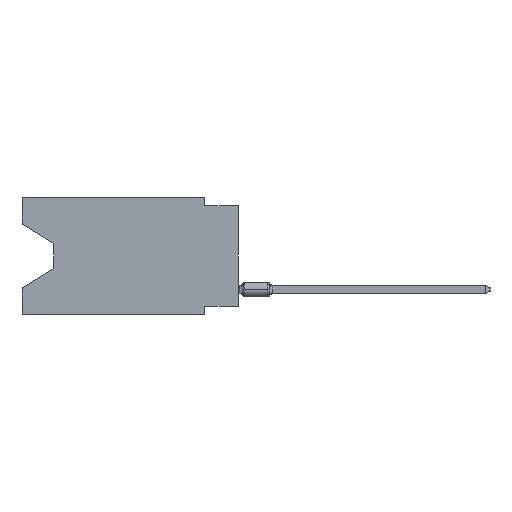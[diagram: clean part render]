
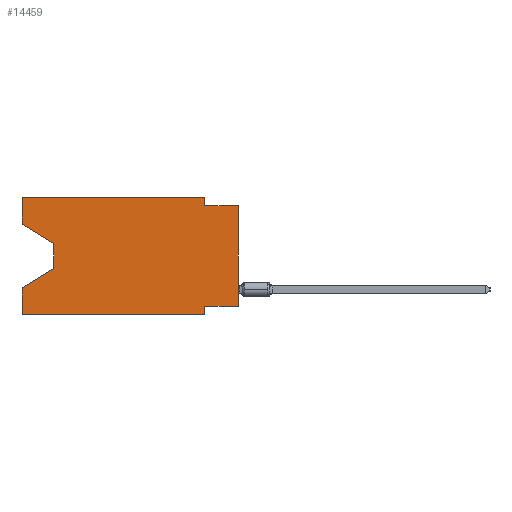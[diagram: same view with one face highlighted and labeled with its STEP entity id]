
A CAD part, left-side view. The second image highlights one B-rep face of the part: STEP entity #14459.
In plain terms, the highlighted planar face has unit normal (-1, 0, 0).
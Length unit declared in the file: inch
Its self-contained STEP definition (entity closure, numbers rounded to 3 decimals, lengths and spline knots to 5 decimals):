
#337 = CARTESIAN_POINT ( 'NONE',  ( 0., 0., -0.325 ) ) ;
#362 = VERTEX_POINT ( 'NONE', #9752 ) ;
#591 = VECTOR ( 'NONE', #44766, 39.37008 ) ;
#774 = CARTESIAN_POINT ( 'NONE',  ( 0., 0., -0.025 ) ) ;
#1442 = VECTOR ( 'NONE', #28018, 39.37008 ) ;
#1944 = ORIENTED_EDGE ( 'NONE', *, *, #45231, .F. ) ;
#2116 = AXIS2_PLACEMENT_3D ( 'NONE', #19843, #26603, #19621 ) ;
#2626 = VECTOR ( 'NONE', #33561, 39.37008 ) ;
#2819 = CARTESIAN_POINT ( 'NONE',  ( 0., 0.55, -0.138 ) ) ;
#3111 = ORIENTED_EDGE ( 'NONE', *, *, #26952, .F. ) ;
#3164 = VECTOR ( 'NONE', #10045, 39.37008 ) ;
#3752 = VERTEX_POINT ( 'NONE', #2819 ) ;
#5478 = ORIENTED_EDGE ( 'NONE', *, *, #40835, .T. ) ;
#5679 = PLANE ( 'NONE',  #2116 ) ;
#6132 = FACE_OUTER_BOUND ( 'NONE', #6671, .T. ) ;
#6144 = CARTESIAN_POINT ( 'NONE',  ( 0., 0., 0. ) ) ;
#6322 = EDGE_CURVE ( 'NONE', #36240, #7142, #17502, .T. ) ;
#6671 = EDGE_LOOP ( 'NONE', ( #13034, #44994, #35203, #3111, #5478, #38925, #16102, #21252, #15470, #29379, #1944, #29011 ) ) ;
#7032 = VERTEX_POINT ( 'NONE', #10753 ) ;
#7142 = VERTEX_POINT ( 'NONE', #774 ) ;
#7881 = VECTOR ( 'NONE', #20769, 39.37008 ) ;
#8308 = LINE ( 'NONE', #36684, #13672 ) ;
#8910 = CARTESIAN_POINT ( 'NONE',  ( 0., 0.55, -0.138 ) ) ;
#9699 = CARTESIAN_POINT ( 'NONE',  ( 0., 0.1, 0. ) ) ;
#9752 = CARTESIAN_POINT ( 'NONE',  ( 0., 0.645, -0.35 ) ) ;
#10045 = DIRECTION ( 'NONE',  ( 0., 0.855, -0.519 ) ) ;
#10753 = CARTESIAN_POINT ( 'NONE',  ( 0., 0.1, -0.025 ) ) ;
#10934 = LINE ( 'NONE', #37156, #29182 ) ;
#10950 = VECTOR ( 'NONE', #18762, 39.37008 ) ;
#11031 = DIRECTION ( 'NONE',  ( 0., 0., 1. ) ) ;
#11550 = LINE ( 'NONE', #29010, #10950 ) ;
#12485 = DIRECTION ( 'NONE',  ( 0., 0., -1. ) ) ;
#13034 = ORIENTED_EDGE ( 'NONE', *, *, #34110, .T. ) ;
#13130 = EDGE_CURVE ( 'NONE', #15213, #35680, #25217, .T. ) ;
#13624 = CARTESIAN_POINT ( 'NONE',  ( 0., 0.645, -0.35 ) ) ;
#13672 = VECTOR ( 'NONE', #25984, 39.37008 ) ;
#14065 = CARTESIAN_POINT ( 'NONE',  ( 0., 0., -0.325 ) ) ;
#14459 = ADVANCED_FACE ( 'NONE', ( #6132 ), #5679, .F. ) ;
#15177 = LINE ( 'NONE', #8910, #2626 ) ;
#15213 = VERTEX_POINT ( 'NONE', #26420 ) ;
#15470 = ORIENTED_EDGE ( 'NONE', *, *, #18663, .F. ) ;
#16076 = LINE ( 'NONE', #44230, #25822 ) ;
#16102 = ORIENTED_EDGE ( 'NONE', *, *, #35900, .F. ) ;
#17017 = LINE ( 'NONE', #27714, #3164 ) ;
#17502 = LINE ( 'NONE', #6144, #7881 ) ;
#18159 = CARTESIAN_POINT ( 'NONE',  ( 0., 0.1, -0.35 ) ) ;
#18237 = LINE ( 'NONE', #14065, #1442 ) ;
#18663 = EDGE_CURVE ( 'NONE', #7032, #7142, #8308, .T. ) ;
#18728 = VECTOR ( 'NONE', #11031, 39.37008 ) ;
#18762 = DIRECTION ( 'NONE',  ( 0., -0.855, -0.519 ) ) ;
#18986 = CARTESIAN_POINT ( 'NONE',  ( 0., 0.645, 0. ) ) ;
#19104 = DIRECTION ( 'NONE',  ( 0., -1., 0. ) ) ;
#19621 = DIRECTION ( 'NONE',  ( 0., 0., -1. ) ) ;
#19843 = CARTESIAN_POINT ( 'NONE',  ( 0., 0.645, 0. ) ) ;
#20078 = VERTEX_POINT ( 'NONE', #23554 ) ;
#20769 = DIRECTION ( 'NONE',  ( 0., 0., 1. ) ) ;
#21252 = ORIENTED_EDGE ( 'NONE', *, *, #6322, .T. ) ;
#23001 = VECTOR ( 'NONE', #28398, 39.37008 ) ;
#23168 = EDGE_CURVE ( 'NONE', #30504, #20078, #17017, .T. ) ;
#23554 = CARTESIAN_POINT ( 'NONE',  ( 0., 0.645, -0.26975 ) ) ;
#25217 = LINE ( 'NONE', #29391, #18728 ) ;
#25822 = VECTOR ( 'NONE', #19104, 39.37008 ) ;
#25984 = DIRECTION ( 'NONE',  ( 0., -1., 0. ) ) ;
#26420 = CARTESIAN_POINT ( 'NONE',  ( 0., 0.645, -0.08025 ) ) ;
#26512 = CARTESIAN_POINT ( 'NONE',  ( 0., 0.55, -0.212 ) ) ;
#26603 = DIRECTION ( 'NONE',  ( 1., 0., 0. ) ) ;
#26952 = EDGE_CURVE ( 'NONE', #362, #20078, #30561, .T. ) ;
#27352 = LINE ( 'NONE', #13624, #33669 ) ;
#27714 = CARTESIAN_POINT ( 'NONE',  ( 0., 0.55, -0.212 ) ) ;
#28018 = DIRECTION ( 'NONE',  ( 0., 1., 0. ) ) ;
#28398 = DIRECTION ( 'NONE',  ( 0., 0., -1. ) ) ;
#29010 = CARTESIAN_POINT ( 'NONE',  ( 0., 0.645, -0.08025 ) ) ;
#29011 = ORIENTED_EDGE ( 'NONE', *, *, #13130, .F. ) ;
#29182 = VECTOR ( 'NONE', #12485, 39.37008 ) ;
#29379 = ORIENTED_EDGE ( 'NONE', *, *, #40695, .F. ) ;
#29391 = CARTESIAN_POINT ( 'NONE',  ( 0., 0.645, 0. ) ) ;
#30504 = VERTEX_POINT ( 'NONE', #26512 ) ;
#30561 = LINE ( 'NONE', #45226, #591 ) ;
#31239 = EDGE_CURVE ( 'NONE', #3752, #30504, #15177, .T. ) ;
#31698 = CARTESIAN_POINT ( 'NONE',  ( 0., 0.1, -0.325 ) ) ;
#33561 = DIRECTION ( 'NONE',  ( 0., 0., -1. ) ) ;
#33669 = VECTOR ( 'NONE', #41095, 39.37008 ) ;
#34110 = EDGE_CURVE ( 'NONE', #15213, #3752, #11550, .T. ) ;
#35203 = ORIENTED_EDGE ( 'NONE', *, *, #23168, .T. ) ;
#35680 = VERTEX_POINT ( 'NONE', #18986 ) ;
#35900 = EDGE_CURVE ( 'NONE', #36240, #41404, #18237, .T. ) ;
#36093 = LINE ( 'NONE', #18159, #23001 ) ;
#36240 = VERTEX_POINT ( 'NONE', #337 ) ;
#36680 = EDGE_CURVE ( 'NONE', #41404, #39321, #36093, .T. ) ;
#36684 = CARTESIAN_POINT ( 'NONE',  ( 0., 0., -0.025 ) ) ;
#37156 = CARTESIAN_POINT ( 'NONE',  ( 0., 0.1, 0. ) ) ;
#38009 = CARTESIAN_POINT ( 'NONE',  ( 0., 0.1, -0.35 ) ) ;
#38885 = VERTEX_POINT ( 'NONE', #9699 ) ;
#38925 = ORIENTED_EDGE ( 'NONE', *, *, #36680, .F. ) ;
#39321 = VERTEX_POINT ( 'NONE', #38009 ) ;
#40695 = EDGE_CURVE ( 'NONE', #38885, #7032, #10934, .T. ) ;
#40835 = EDGE_CURVE ( 'NONE', #362, #39321, #27352, .T. ) ;
#41095 = DIRECTION ( 'NONE',  ( 0., -1., 0. ) ) ;
#41404 = VERTEX_POINT ( 'NONE', #31698 ) ;
#44230 = CARTESIAN_POINT ( 'NONE',  ( 0., 0.645, 0. ) ) ;
#44766 = DIRECTION ( 'NONE',  ( 0., 0., 1. ) ) ;
#44994 = ORIENTED_EDGE ( 'NONE', *, *, #31239, .T. ) ;
#45226 = CARTESIAN_POINT ( 'NONE',  ( 0., 0.645, 0. ) ) ;
#45231 = EDGE_CURVE ( 'NONE', #35680, #38885, #16076, .T. ) ;
